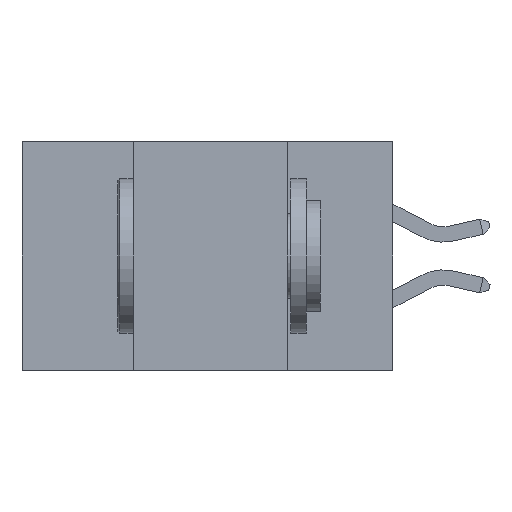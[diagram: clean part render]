
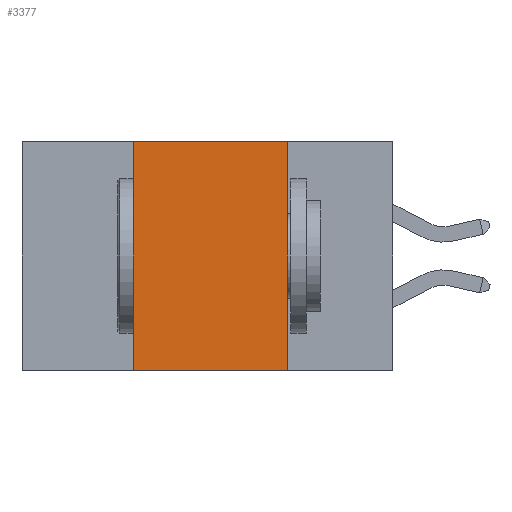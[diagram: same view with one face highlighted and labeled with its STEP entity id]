
A CAD part, left-side view. The second image highlights one B-rep face of the part: STEP entity #3377.
In plain terms, the highlighted planar face has unit normal (-1, 0, 0).
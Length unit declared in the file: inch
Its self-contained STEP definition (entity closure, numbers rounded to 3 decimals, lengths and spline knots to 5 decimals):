
#1359 = DIRECTION ( 'NONE',  ( 0., -1., 0. ) ) ;
#2226 = DIRECTION ( 'NONE',  ( 0., 0., 1. ) ) ;
#2851 = PLANE ( 'NONE',  #9590 ) ;
#3377 = ADVANCED_FACE ( 'NONE', ( #11076 ), #2851, .F. ) ;
#3817 = CARTESIAN_POINT ( 'NONE',  ( 0., 0.42, -0.37 ) ) ;
#4190 = VECTOR ( 'NONE', #10928, 39.37008 ) ;
#4605 = LINE ( 'NONE', #7040, #13045 ) ;
#5403 = DIRECTION ( 'NONE',  ( 1., 0., 0. ) ) ;
#6111 = CARTESIAN_POINT ( 'NONE',  ( 0., 0.6, 0. ) ) ;
#6226 = DIRECTION ( 'NONE',  ( 0., 0., -1. ) ) ;
#6312 = CARTESIAN_POINT ( 'NONE',  ( 0., 0.6, 0. ) ) ;
#6403 = LINE ( 'NONE', #10533, #14264 ) ;
#6791 = VERTEX_POINT ( 'NONE', #13610 ) ;
#6944 = CARTESIAN_POINT ( 'NONE',  ( 0., 0.42, 0. ) ) ;
#7040 = CARTESIAN_POINT ( 'NONE',  ( 0., 0.42, 0. ) ) ;
#7110 = VERTEX_POINT ( 'NONE', #3817 ) ;
#7142 = EDGE_CURVE ( 'NONE', #8718, #7445, #12151, .T. ) ;
#7445 = VERTEX_POINT ( 'NONE', #7987 ) ;
#7585 = EDGE_CURVE ( 'NONE', #7445, #6791, #6403, .T. ) ;
#7819 = ORIENTED_EDGE ( 'NONE', *, *, #7585, .F. ) ;
#7987 = CARTESIAN_POINT ( 'NONE',  ( 0., 0.17, 0. ) ) ;
#8718 = VERTEX_POINT ( 'NONE', #6944 ) ;
#9590 = AXIS2_PLACEMENT_3D ( 'NONE', #6111, #5403, #6226 ) ;
#9760 = CARTESIAN_POINT ( 'NONE',  ( 0., 0.6, -0.37 ) ) ;
#10022 = EDGE_LOOP ( 'NONE', ( #7819, #10871, #13740, #11238 ) ) ;
#10414 = LINE ( 'NONE', #9760, #4190 ) ;
#10533 = CARTESIAN_POINT ( 'NONE',  ( 0., 0.17, 0. ) ) ;
#10871 = ORIENTED_EDGE ( 'NONE', *, *, #7142, .F. ) ;
#10928 = DIRECTION ( 'NONE',  ( 0., -1., 0. ) ) ;
#11076 = FACE_OUTER_BOUND ( 'NONE', #10022, .T. ) ;
#11238 = ORIENTED_EDGE ( 'NONE', *, *, #14738, .T. ) ;
#12151 = LINE ( 'NONE', #6312, #14279 ) ;
#12780 = DIRECTION ( 'NONE',  ( 0., 0., -1. ) ) ;
#13045 = VECTOR ( 'NONE', #2226, 39.37008 ) ;
#13610 = CARTESIAN_POINT ( 'NONE',  ( 0., 0.17, -0.37 ) ) ;
#13740 = ORIENTED_EDGE ( 'NONE', *, *, #13924, .F. ) ;
#13924 = EDGE_CURVE ( 'NONE', #7110, #8718, #4605, .T. ) ;
#14264 = VECTOR ( 'NONE', #12780, 39.37008 ) ;
#14279 = VECTOR ( 'NONE', #1359, 39.37008 ) ;
#14738 = EDGE_CURVE ( 'NONE', #7110, #6791, #10414, .T. ) ;
